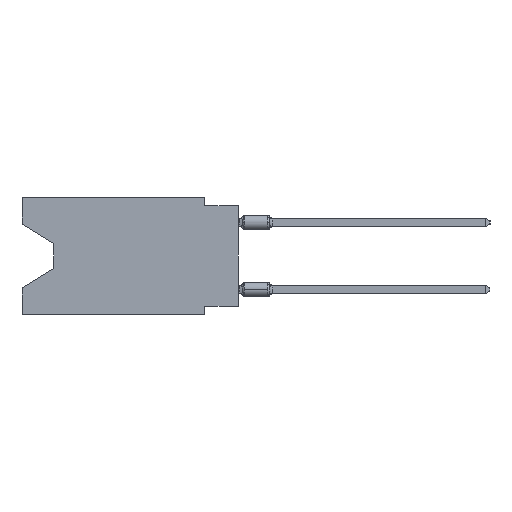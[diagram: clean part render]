
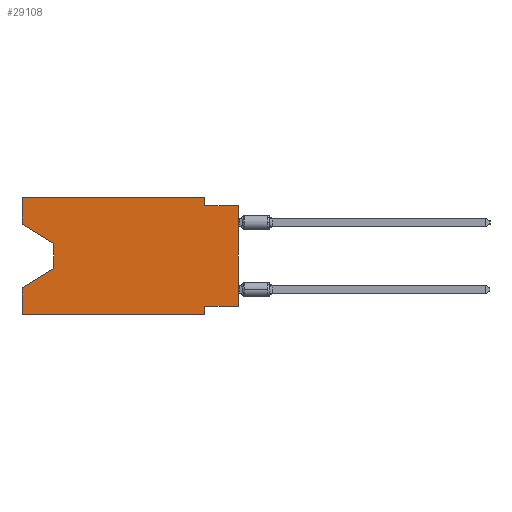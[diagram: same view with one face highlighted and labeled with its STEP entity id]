
A CAD part, left-side view. The second image highlights one B-rep face of the part: STEP entity #29108.
In plain terms, the highlighted planar face has unit normal (-1, 0, 0).
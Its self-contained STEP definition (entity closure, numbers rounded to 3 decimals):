
#1799 = VERTEX_POINT ( 'NONE', #20928 ) ;
#2299 = ORIENTED_EDGE ( 'NONE', *, *, #4901, .T. ) ;
#2920 = EDGE_CURVE ( 'NONE', #4341, #18197, #10472, .T. ) ;
#3799 = CARTESIAN_POINT ( 'NONE',  ( 0., 2.54, -0.635 ) ) ;
#4341 = VERTEX_POINT ( 'NONE', #7739 ) ;
#4600 = EDGE_CURVE ( 'NONE', #16526, #45688, #30740, .T. ) ;
#4901 = EDGE_CURVE ( 'NONE', #38920, #1799, #40867, .T. ) ;
#6051 = ORIENTED_EDGE ( 'NONE', *, *, #13208, .F. ) ;
#6517 = DIRECTION ( 'NONE',  ( 0., -0.855, -0.519 ) ) ;
#6614 = DIRECTION ( 'NONE',  ( 1., 0., 0. ) ) ;
#6920 = VECTOR ( 'NONE', #8381, 1000. ) ;
#7728 = VERTEX_POINT ( 'NONE', #37732 ) ;
#7739 = CARTESIAN_POINT ( 'NONE',  ( 0., 16.383, -2.038 ) ) ;
#7955 = EDGE_CURVE ( 'NONE', #41661, #7728, #43299, .T. ) ;
#8381 = DIRECTION ( 'NONE',  ( 0., 0., -1. ) ) ;
#8758 = CARTESIAN_POINT ( 'NONE',  ( 0., 16.383, 0. ) ) ;
#9123 = LINE ( 'NONE', #33801, #13947 ) ;
#9363 = DIRECTION ( 'NONE',  ( 0., 0., -1. ) ) ;
#9636 = FACE_OUTER_BOUND ( 'NONE', #35707, .T. ) ;
#9831 = VECTOR ( 'NONE', #11649, 1000. ) ;
#9852 = EDGE_CURVE ( 'NONE', #38920, #16526, #16244, .T. ) ;
#10472 = LINE ( 'NONE', #14428, #42357 ) ;
#10816 = VECTOR ( 'NONE', #29948, 1000. ) ;
#11437 = EDGE_CURVE ( 'NONE', #4341, #42185, #19241, .T. ) ;
#11649 = DIRECTION ( 'NONE',  ( 0., 0.855, -0.519 ) ) ;
#12329 = CARTESIAN_POINT ( 'NONE',  ( 0., 13.97, -5.385 ) ) ;
#12540 = CARTESIAN_POINT ( 'NONE',  ( 0., 16.383, 0. ) ) ;
#13208 = EDGE_CURVE ( 'NONE', #18862, #7728, #45213, .T. ) ;
#13356 = PLANE ( 'NONE',  #43772 ) ;
#13558 = CARTESIAN_POINT ( 'NONE',  ( 0., 16.383, 0. ) ) ;
#13734 = DIRECTION ( 'NONE',  ( 0., 0., -1. ) ) ;
#13874 = ORIENTED_EDGE ( 'NONE', *, *, #39692, .F. ) ;
#13947 = VECTOR ( 'NONE', #19615, 1000. ) ;
#14428 = CARTESIAN_POINT ( 'NONE',  ( 0., 16.383, -2.038 ) ) ;
#15260 = ORIENTED_EDGE ( 'NONE', *, *, #11437, .F. ) ;
#15592 = CARTESIAN_POINT ( 'NONE',  ( 0., 13.97, -3.505 ) ) ;
#15706 = EDGE_CURVE ( 'NONE', #35740, #37310, #45196, .T. ) ;
#16228 = DIRECTION ( 'NONE',  ( 0., -1., 0. ) ) ;
#16244 = LINE ( 'NONE', #44169, #32971 ) ;
#16526 = VERTEX_POINT ( 'NONE', #24561 ) ;
#17994 = ORIENTED_EDGE ( 'NONE', *, *, #2920, .T. ) ;
#18197 = VERTEX_POINT ( 'NONE', #18641 ) ;
#18641 = CARTESIAN_POINT ( 'NONE',  ( 0., 13.97, -3.505 ) ) ;
#18862 = VERTEX_POINT ( 'NONE', #24835 ) ;
#18928 = VECTOR ( 'NONE', #16228, 1000. ) ;
#19241 = LINE ( 'NONE', #8758, #10816 ) ;
#19248 = CARTESIAN_POINT ( 'NONE',  ( 0., 0., 0. ) ) ;
#19615 = DIRECTION ( 'NONE',  ( 0., -1., 0. ) ) ;
#20039 = CARTESIAN_POINT ( 'NONE',  ( 0., 2.54, -8.89 ) ) ;
#20127 = CARTESIAN_POINT ( 'NONE',  ( 0., 16.383, 0. ) ) ;
#20559 = CARTESIAN_POINT ( 'NONE',  ( 0., 16.383, -8.89 ) ) ;
#20928 = CARTESIAN_POINT ( 'NONE',  ( 0., 0., -0.635 ) ) ;
#22005 = VECTOR ( 'NONE', #31959, 1000. ) ;
#22732 = DIRECTION ( 'NONE',  ( 0., 0., 1. ) ) ;
#23178 = VECTOR ( 'NONE', #45683, 1000. ) ;
#23431 = ORIENTED_EDGE ( 'NONE', *, *, #25684, .T. ) ;
#24311 = DIRECTION ( 'NONE',  ( 0., 0., -1. ) ) ;
#24561 = CARTESIAN_POINT ( 'NONE',  ( 0., 2.54, -8.255 ) ) ;
#24835 = CARTESIAN_POINT ( 'NONE',  ( 0., 16.383, -8.89 ) ) ;
#25615 = VECTOR ( 'NONE', #9363, 1000. ) ;
#25684 = EDGE_CURVE ( 'NONE', #18197, #41661, #26935, .T. ) ;
#25840 = VECTOR ( 'NONE', #13734, 1000. ) ;
#26935 = LINE ( 'NONE', #15592, #6920 ) ;
#27188 = DIRECTION ( 'NONE',  ( 0., 1., 0. ) ) ;
#27743 = CARTESIAN_POINT ( 'NONE',  ( 0., 0., -8.255 ) ) ;
#27783 = EDGE_CURVE ( 'NONE', #37310, #1799, #9123, .T. ) ;
#29108 = ADVANCED_FACE ( 'NONE', ( #9636 ), #13356, .F. ) ;
#29948 = DIRECTION ( 'NONE',  ( 0., 0., 1. ) ) ;
#30740 = LINE ( 'NONE', #20039, #25840 ) ;
#31959 = DIRECTION ( 'NONE',  ( 0., -1., 0. ) ) ;
#32971 = VECTOR ( 'NONE', #27188, 1000. ) ;
#33801 = CARTESIAN_POINT ( 'NONE',  ( 0., 0., -0.635 ) ) ;
#34229 = ORIENTED_EDGE ( 'NONE', *, *, #27783, .F. ) ;
#34519 = EDGE_CURVE ( 'NONE', #18862, #45688, #41965, .T. ) ;
#35465 = CARTESIAN_POINT ( 'NONE',  ( 0., 2.54, 0. ) ) ;
#35707 = EDGE_LOOP ( 'NONE', ( #17994, #23431, #45121, #6051, #36757, #42366, #35886, #2299, #34229, #43103, #13874, #15260 ) ) ;
#35740 = VERTEX_POINT ( 'NONE', #35465 ) ;
#35886 = ORIENTED_EDGE ( 'NONE', *, *, #9852, .F. ) ;
#36757 = ORIENTED_EDGE ( 'NONE', *, *, #34519, .T. ) ;
#37123 = CARTESIAN_POINT ( 'NONE',  ( 0., 2.54, -8.89 ) ) ;
#37310 = VERTEX_POINT ( 'NONE', #3799 ) ;
#37732 = CARTESIAN_POINT ( 'NONE',  ( 0., 16.383, -6.852 ) ) ;
#37979 = CARTESIAN_POINT ( 'NONE',  ( 0., 2.54, 0. ) ) ;
#38920 = VERTEX_POINT ( 'NONE', #27743 ) ;
#39692 = EDGE_CURVE ( 'NONE', #42185, #35740, #44599, .T. ) ;
#40867 = LINE ( 'NONE', #19248, #41460 ) ;
#41121 = CARTESIAN_POINT ( 'NONE',  ( 0., 16.383, 0. ) ) ;
#41460 = VECTOR ( 'NONE', #22732, 1000. ) ;
#41661 = VERTEX_POINT ( 'NONE', #45744 ) ;
#41965 = LINE ( 'NONE', #20559, #22005 ) ;
#42185 = VERTEX_POINT ( 'NONE', #12540 ) ;
#42357 = VECTOR ( 'NONE', #6517, 1000. ) ;
#42366 = ORIENTED_EDGE ( 'NONE', *, *, #4600, .F. ) ;
#43103 = ORIENTED_EDGE ( 'NONE', *, *, #15706, .F. ) ;
#43299 = LINE ( 'NONE', #12329, #9831 ) ;
#43772 = AXIS2_PLACEMENT_3D ( 'NONE', #20127, #6614, #24311 ) ;
#44169 = CARTESIAN_POINT ( 'NONE',  ( 0., 0., -8.255 ) ) ;
#44599 = LINE ( 'NONE', #41121, #18928 ) ;
#45121 = ORIENTED_EDGE ( 'NONE', *, *, #7955, .T. ) ;
#45196 = LINE ( 'NONE', #37979, #25615 ) ;
#45213 = LINE ( 'NONE', #13558, #23178 ) ;
#45683 = DIRECTION ( 'NONE',  ( 0., 0., 1. ) ) ;
#45688 = VERTEX_POINT ( 'NONE', #37123 ) ;
#45744 = CARTESIAN_POINT ( 'NONE',  ( 0., 13.97, -5.385 ) ) ;
